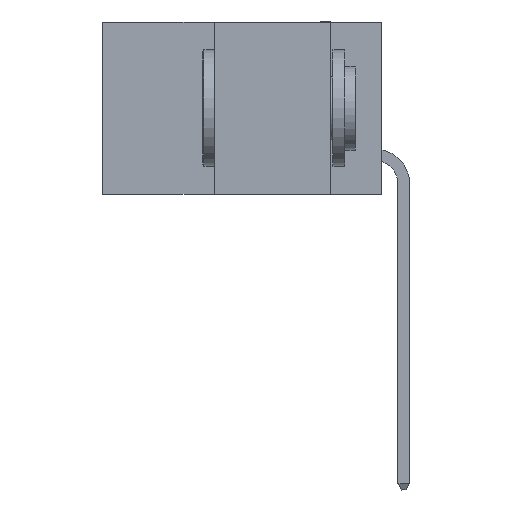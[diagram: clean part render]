
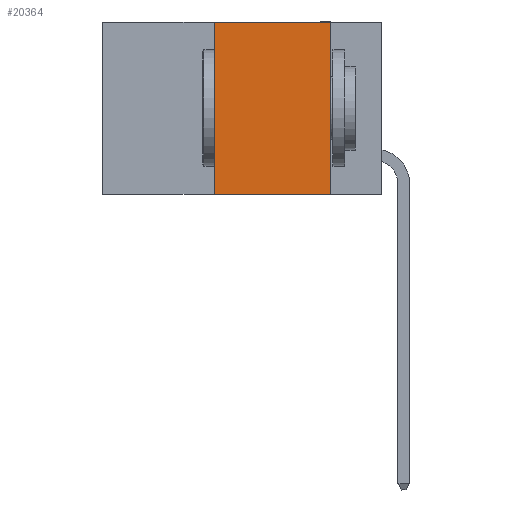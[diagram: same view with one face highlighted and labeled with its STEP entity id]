
A CAD part, left-side view. The second image highlights one B-rep face of the part: STEP entity #20364.
In plain terms, the highlighted planar face has unit normal (-1, 0, 0).
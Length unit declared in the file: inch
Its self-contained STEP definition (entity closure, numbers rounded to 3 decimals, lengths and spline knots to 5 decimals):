
#1757 = VECTOR ( 'NONE', #13489, 39.37008 ) ;
#2820 = CARTESIAN_POINT ( 'NONE',  ( 0., 0.6, 0. ) ) ;
#3862 = AXIS2_PLACEMENT_3D ( 'NONE', #2820, #12258, #28736 ) ;
#4825 = CARTESIAN_POINT ( 'NONE',  ( 0., 0.36, -0.37 ) ) ;
#7591 = LINE ( 'NONE', #21150, #13023 ) ;
#7879 = CARTESIAN_POINT ( 'NONE',  ( 0., 0.36, 0. ) ) ;
#8340 = DIRECTION ( 'NONE',  ( 0., 0., 1. ) ) ;
#9155 = VERTEX_POINT ( 'NONE', #4825 ) ;
#9450 = DIRECTION ( 'NONE',  ( 0., -1., 0. ) ) ;
#9778 = LINE ( 'NONE', #16390, #21539 ) ;
#9927 = PLANE ( 'NONE',  #3862 ) ;
#10186 = VERTEX_POINT ( 'NONE', #29770 ) ;
#10356 = VERTEX_POINT ( 'NONE', #30269 ) ;
#12258 = DIRECTION ( 'NONE',  ( 1., 0., 0. ) ) ;
#13023 = VECTOR ( 'NONE', #9450, 39.37008 ) ;
#13489 = DIRECTION ( 'NONE',  ( 0., 0., -1. ) ) ;
#13659 = LINE ( 'NONE', #24771, #19154 ) ;
#14388 = EDGE_CURVE ( 'NONE', #10186, #10356, #20546, .T. ) ;
#15638 = EDGE_CURVE ( 'NONE', #27359, #10186, #7591, .T. ) ;
#16224 = EDGE_LOOP ( 'NONE', ( #30038, #28216, #23441, #21597 ) ) ;
#16390 = CARTESIAN_POINT ( 'NONE',  ( 0., 0.6, -0.37 ) ) ;
#18057 = EDGE_CURVE ( 'NONE', #9155, #27359, #13659, .T. ) ;
#19154 = VECTOR ( 'NONE', #8340, 39.37008 ) ;
#20364 = ADVANCED_FACE ( 'NONE', ( #21626 ), #9927, .F. ) ;
#20546 = LINE ( 'NONE', #22884, #1757 ) ;
#21150 = CARTESIAN_POINT ( 'NONE',  ( 0., 0.6, 0. ) ) ;
#21539 = VECTOR ( 'NONE', #28231, 39.37008 ) ;
#21597 = ORIENTED_EDGE ( 'NONE', *, *, #23452, .T. ) ;
#21626 = FACE_OUTER_BOUND ( 'NONE', #16224, .T. ) ;
#22884 = CARTESIAN_POINT ( 'NONE',  ( 0., 0.11, 0. ) ) ;
#23441 = ORIENTED_EDGE ( 'NONE', *, *, #18057, .F. ) ;
#23452 = EDGE_CURVE ( 'NONE', #9155, #10356, #9778, .T. ) ;
#24771 = CARTESIAN_POINT ( 'NONE',  ( 0., 0.36, 0. ) ) ;
#27359 = VERTEX_POINT ( 'NONE', #7879 ) ;
#28216 = ORIENTED_EDGE ( 'NONE', *, *, #15638, .F. ) ;
#28231 = DIRECTION ( 'NONE',  ( 0., -1., 0. ) ) ;
#28736 = DIRECTION ( 'NONE',  ( 0., 0., -1. ) ) ;
#29770 = CARTESIAN_POINT ( 'NONE',  ( 0., 0.11, 0. ) ) ;
#30038 = ORIENTED_EDGE ( 'NONE', *, *, #14388, .F. ) ;
#30269 = CARTESIAN_POINT ( 'NONE',  ( 0., 0.11, -0.37 ) ) ;
